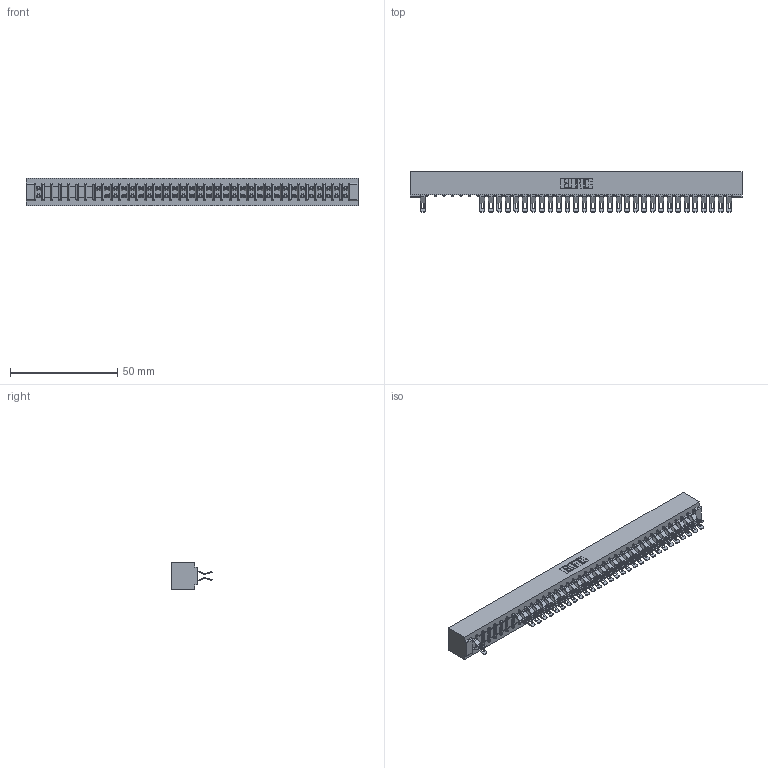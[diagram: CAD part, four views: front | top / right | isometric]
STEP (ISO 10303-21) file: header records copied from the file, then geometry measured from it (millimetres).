
FILE_DESCRIPTION (( 'STEP AP203' ), '1' );
FILE_NAME ('307-074-555-201.STEP', '2018-08-06T16:18:20', ( '' ), ( '' ), 'SwSTEP 2.0', 'SolidWorks 2016', '' );
FILE_SCHEMA (( 'CONFIG_CONTROL_DESIGN' ));
Length unit declared in the file: inch
Products named in the file (3): 307-290-001_555; 307-074-555-201; 307 Part_No Mounting Lugs
Assembly tree (62 placements, depth 2):
  307-074-555-201
    307 Part_No Mounting Lugs
    307-290-001_555  x61
Bounding box: 154.48 x 18.75 x 12.7 mm (x, y, z)
Volume: 16953 mm3; surface area: 20860.4 mm2
Topology: 62 solids, 62 shells, 3999 faces, 11756 edges, 7652 vertices
Faces by surface type: plane 2218, cylinder 1705, sphere 76
Entity records: 33363 total; most frequent: CARTESIAN_POINT 5516, ORIENTED_EDGE 5480, DIRECTION 5398, EDGE_CURVE 2740, LINE 2090, VECTOR 2090, VERTEX_POINT 1772, AXIS2_PLACEMENT_3D 1654
